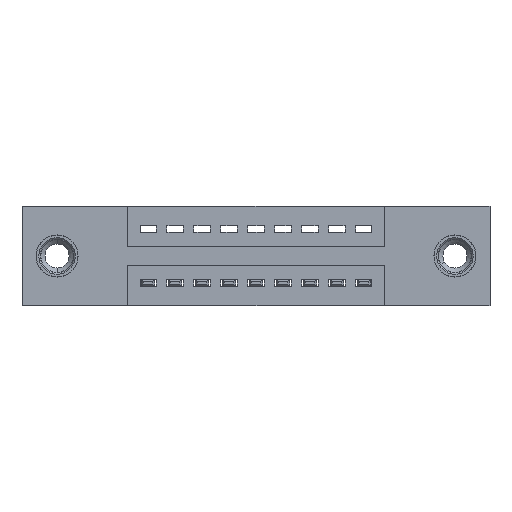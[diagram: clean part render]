
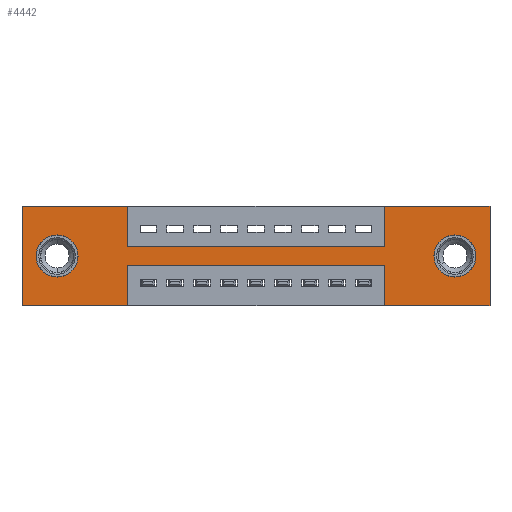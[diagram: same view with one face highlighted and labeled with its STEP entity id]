
A CAD part, front view. The second image highlights one B-rep face of the part: STEP entity #4442.
In plain terms, the highlighted planar face has unit normal (0, -1, 0).
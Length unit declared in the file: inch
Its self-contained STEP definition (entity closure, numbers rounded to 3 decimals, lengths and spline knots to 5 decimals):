
#3 = DIRECTION ( 'NONE',  ( 0., 1., 0. ) ) ;
#271 = ORIENTED_EDGE ( 'NONE', *, *, #3177, .T. ) ;
#413 = VERTEX_POINT ( 'NONE', #10230 ) ;
#442 = ORIENTED_EDGE ( 'NONE', *, *, #7183, .F. ) ;
#518 = CARTESIAN_POINT ( 'NONE',  ( 0.3925, 0., -0.37 ) ) ;
#746 = EDGE_CURVE ( 'NONE', #2080, #7335, #2838, .T. ) ;
#867 = DIRECTION ( 'NONE',  ( 1., 0., 0. ) ) ;
#895 = DIRECTION ( 'NONE',  ( 0., 0., -1. ) ) ;
#913 = ORIENTED_EDGE ( 'NONE', *, *, #9199, .F. ) ;
#1053 = CARTESIAN_POINT ( 'NONE',  ( 0., 0., 0. ) ) ;
#1136 = LINE ( 'NONE', #2850, #7727 ) ;
#1156 = CARTESIAN_POINT ( 'NONE',  ( 1.3425, 0., -0.15 ) ) ;
#1185 = ORIENTED_EDGE ( 'NONE', *, *, #5416, .F. ) ;
#1276 = CARTESIAN_POINT ( 'NONE',  ( 0.13, 0., -0.107 ) ) ;
#1354 = ORIENTED_EDGE ( 'NONE', *, *, #1799, .T. ) ;
#1493 = VECTOR ( 'NONE', #5650, 39.37008 ) ;
#1651 = DIRECTION ( 'NONE',  ( -1., 0., 0. ) ) ;
#1770 = CARTESIAN_POINT ( 'NONE',  ( 0.3925, 0., -0.22 ) ) ;
#1799 = EDGE_CURVE ( 'NONE', #8598, #413, #11335, .T. ) ;
#1884 = PLANE ( 'NONE',  #5999 ) ;
#1992 = DIRECTION ( 'NONE',  ( 1., 0., 0. ) ) ;
#2080 = VERTEX_POINT ( 'NONE', #1156 ) ;
#2261 = VERTEX_POINT ( 'NONE', #11005 ) ;
#2326 = CARTESIAN_POINT ( 'NONE',  ( 1.3425, 0., 0. ) ) ;
#2395 = EDGE_CURVE ( 'NONE', #7335, #11135, #8940, .T. ) ;
#2505 = ORIENTED_EDGE ( 'NONE', *, *, #2395, .F. ) ;
#2549 = DIRECTION ( 'NONE',  ( 0., 1., 0. ) ) ;
#2581 = AXIS2_PLACEMENT_3D ( 'NONE', #9398, #3808, #8330 ) ;
#2606 = VERTEX_POINT ( 'NONE', #7716 ) ;
#2838 = LINE ( 'NONE', #9803, #11215 ) ;
#2850 = CARTESIAN_POINT ( 'NONE',  ( 0.3925, 0., -0.37 ) ) ;
#2995 = CARTESIAN_POINT ( 'NONE',  ( 0.3925, 0., -0.15 ) ) ;
#3018 = CARTESIAN_POINT ( 'NONE',  ( 0.3925, 0., -0.22 ) ) ;
#3069 = VERTEX_POINT ( 'NONE', #1276 ) ;
#3105 = EDGE_CURVE ( 'NONE', #11135, #5520, #8944, .T. ) ;
#3177 = EDGE_CURVE ( 'NONE', #413, #8598, #6465, .T. ) ;
#3185 = ORIENTED_EDGE ( 'NONE', *, *, #3105, .F. ) ;
#3366 = CARTESIAN_POINT ( 'NONE',  ( 1.735, 0., -0.37 ) ) ;
#3478 = CARTESIAN_POINT ( 'NONE',  ( 1.3425, 0., -0.37 ) ) ;
#3547 = LINE ( 'NONE', #10758, #9218 ) ;
#3614 = ORIENTED_EDGE ( 'NONE', *, *, #11353, .F. ) ;
#3808 = DIRECTION ( 'NONE',  ( 0., 1., 0. ) ) ;
#3964 = DIRECTION ( 'NONE',  ( 0., 0., -1. ) ) ;
#3978 = EDGE_CURVE ( 'NONE', #4640, #4697, #9960, .T. ) ;
#4180 = AXIS2_PLACEMENT_3D ( 'NONE', #11761, #2549, #10909 ) ;
#4350 = VECTOR ( 'NONE', #1992, 39.37008 ) ;
#4442 = ADVANCED_FACE ( 'NONE', ( #7151, #11274, #8022 ), #1884, .T. ) ;
#4510 = ORIENTED_EDGE ( 'NONE', *, *, #11435, .F. ) ;
#4640 = VERTEX_POINT ( 'NONE', #8678 ) ;
#4697 = VERTEX_POINT ( 'NONE', #8754 ) ;
#4755 = CIRCLE ( 'NONE', #6246, 0.078 ) ;
#4995 = DIRECTION ( 'NONE',  ( 0., 1., 0. ) ) ;
#5001 = CARTESIAN_POINT ( 'NONE',  ( 0.3925, 0., 0. ) ) ;
#5041 = LINE ( 'NONE', #3478, #9084 ) ;
#5226 = CIRCLE ( 'NONE', #4180, 0.078 ) ;
#5318 = VECTOR ( 'NONE', #867, 39.37008 ) ;
#5327 = LINE ( 'NONE', #10306, #1493 ) ;
#5374 = DIRECTION ( 'NONE',  ( 0., 0., 1. ) ) ;
#5416 = EDGE_CURVE ( 'NONE', #8078, #8844, #10836, .T. ) ;
#5470 = VECTOR ( 'NONE', #11986, 39.37008 ) ;
#5520 = VERTEX_POINT ( 'NONE', #3366 ) ;
#5650 = DIRECTION ( 'NONE',  ( -1., 0., 0. ) ) ;
#5776 = CARTESIAN_POINT ( 'NONE',  ( 0.13, 0., -0.185 ) ) ;
#5940 = CARTESIAN_POINT ( 'NONE',  ( 0.13, 0., -0.263 ) ) ;
#5999 = AXIS2_PLACEMENT_3D ( 'NONE', #12231, #11164, #895 ) ;
#6017 = ORIENTED_EDGE ( 'NONE', *, *, #3978, .F. ) ;
#6239 = DIRECTION ( 'NONE',  ( 0., 0., -1. ) ) ;
#6246 = AXIS2_PLACEMENT_3D ( 'NONE', #5776, #3, #7465 ) ;
#6303 = VECTOR ( 'NONE', #3964, 39.37008 ) ;
#6465 = CIRCLE ( 'NONE', #6916, 0.078 ) ;
#6471 = ORIENTED_EDGE ( 'NONE', *, *, #7476, .T. ) ;
#6772 = VERTEX_POINT ( 'NONE', #7768 ) ;
#6908 = LINE ( 'NONE', #1770, #5470 ) ;
#6916 = AXIS2_PLACEMENT_3D ( 'NONE', #10548, #4995, #6239 ) ;
#7151 = FACE_BOUND ( 'NONE', #9599, .T. ) ;
#7183 = EDGE_CURVE ( 'NONE', #2261, #4640, #9575, .T. ) ;
#7335 = VERTEX_POINT ( 'NONE', #2326 ) ;
#7396 = EDGE_LOOP ( 'NONE', ( #8353, #4510, #3614, #8971, #3185, #2505, #11748, #9164, #6017, #442, #913, #1185 ) ) ;
#7465 = DIRECTION ( 'NONE',  ( 0., 0., 1. ) ) ;
#7476 = EDGE_CURVE ( 'NONE', #10048, #3069, #5226, .T. ) ;
#7692 = CARTESIAN_POINT ( 'NONE',  ( 1.735, 0., 0. ) ) ;
#7716 = CARTESIAN_POINT ( 'NONE',  ( 1.3425, 0., -0.22 ) ) ;
#7727 = VECTOR ( 'NONE', #11229, 39.37008 ) ;
#7768 = CARTESIAN_POINT ( 'NONE',  ( 1.3425, 0., -0.37 ) ) ;
#8022 = FACE_OUTER_BOUND ( 'NONE', #7396, .T. ) ;
#8078 = VERTEX_POINT ( 'NONE', #518 ) ;
#8310 = VECTOR ( 'NONE', #1651, 39.37008 ) ;
#8330 = DIRECTION ( 'NONE',  ( 0., 0., -1. ) ) ;
#8353 = ORIENTED_EDGE ( 'NONE', *, *, #10858, .F. ) ;
#8598 = VERTEX_POINT ( 'NONE', #12132 ) ;
#8678 = CARTESIAN_POINT ( 'NONE',  ( 0.3925, 0., 0. ) ) ;
#8725 = DIRECTION ( 'NONE',  ( 0., 0., 1. ) ) ;
#8744 = ORIENTED_EDGE ( 'NONE', *, *, #11204, .T. ) ;
#8754 = CARTESIAN_POINT ( 'NONE',  ( 0.3925, 0., -0.15 ) ) ;
#8844 = VERTEX_POINT ( 'NONE', #10524 ) ;
#8940 = LINE ( 'NONE', #12092, #5318 ) ;
#8944 = LINE ( 'NONE', #7692, #9237 ) ;
#8971 = ORIENTED_EDGE ( 'NONE', *, *, #11216, .F. ) ;
#9084 = VECTOR ( 'NONE', #5374, 39.37008 ) ;
#9164 = ORIENTED_EDGE ( 'NONE', *, *, #10276, .F. ) ;
#9199 = EDGE_CURVE ( 'NONE', #8844, #2261, #3547, .T. ) ;
#9218 = VECTOR ( 'NONE', #11686, 39.37008 ) ;
#9237 = VECTOR ( 'NONE', #11575, 39.37008 ) ;
#9398 = CARTESIAN_POINT ( 'NONE',  ( 1.605, 0., -0.185 ) ) ;
#9504 = VECTOR ( 'NONE', #10378, 39.37008 ) ;
#9575 = LINE ( 'NONE', #1053, #4350 ) ;
#9599 = EDGE_LOOP ( 'NONE', ( #271, #1354 ) ) ;
#9803 = CARTESIAN_POINT ( 'NONE',  ( 1.3425, 0., 0. ) ) ;
#9960 = LINE ( 'NONE', #5001, #6303 ) ;
#10048 = VERTEX_POINT ( 'NONE', #5940 ) ;
#10230 = CARTESIAN_POINT ( 'NONE',  ( 1.605, 0., -0.107 ) ) ;
#10276 = EDGE_CURVE ( 'NONE', #4697, #2080, #10725, .T. ) ;
#10306 = CARTESIAN_POINT ( 'NONE',  ( 0., 0., -0.37 ) ) ;
#10378 = DIRECTION ( 'NONE',  ( 1., 0., 0. ) ) ;
#10524 = CARTESIAN_POINT ( 'NONE',  ( 0., 0., -0.37 ) ) ;
#10548 = CARTESIAN_POINT ( 'NONE',  ( 1.605, 0., -0.185 ) ) ;
#10725 = LINE ( 'NONE', #2995, #9504 ) ;
#10758 = CARTESIAN_POINT ( 'NONE',  ( 0., 0., 0. ) ) ;
#10836 = LINE ( 'NONE', #10845, #8310 ) ;
#10845 = CARTESIAN_POINT ( 'NONE',  ( 0., 0., -0.37 ) ) ;
#10858 = EDGE_CURVE ( 'NONE', #11000, #8078, #1136, .T. ) ;
#10891 = EDGE_LOOP ( 'NONE', ( #8744, #6471 ) ) ;
#10909 = DIRECTION ( 'NONE',  ( 0., 0., 1. ) ) ;
#10977 = CARTESIAN_POINT ( 'NONE',  ( 1.735, 0., 0. ) ) ;
#11000 = VERTEX_POINT ( 'NONE', #3018 ) ;
#11005 = CARTESIAN_POINT ( 'NONE',  ( 0., 0., 0. ) ) ;
#11135 = VERTEX_POINT ( 'NONE', #10977 ) ;
#11164 = DIRECTION ( 'NONE',  ( 0., -1., 0. ) ) ;
#11204 = EDGE_CURVE ( 'NONE', #3069, #10048, #4755, .T. ) ;
#11215 = VECTOR ( 'NONE', #8725, 39.37008 ) ;
#11216 = EDGE_CURVE ( 'NONE', #5520, #6772, #5327, .T. ) ;
#11229 = DIRECTION ( 'NONE',  ( 0., 0., -1. ) ) ;
#11274 = FACE_BOUND ( 'NONE', #10891, .T. ) ;
#11335 = CIRCLE ( 'NONE', #2581, 0.078 ) ;
#11353 = EDGE_CURVE ( 'NONE', #6772, #2606, #5041, .T. ) ;
#11435 = EDGE_CURVE ( 'NONE', #2606, #11000, #6908, .T. ) ;
#11575 = DIRECTION ( 'NONE',  ( 0., 0., -1. ) ) ;
#11686 = DIRECTION ( 'NONE',  ( 0., 0., 1. ) ) ;
#11748 = ORIENTED_EDGE ( 'NONE', *, *, #746, .F. ) ;
#11761 = CARTESIAN_POINT ( 'NONE',  ( 0.13, 0., -0.185 ) ) ;
#11986 = DIRECTION ( 'NONE',  ( -1., 0., 0. ) ) ;
#12092 = CARTESIAN_POINT ( 'NONE',  ( 0., 0., 0. ) ) ;
#12132 = CARTESIAN_POINT ( 'NONE',  ( 1.605, 0., -0.263 ) ) ;
#12231 = CARTESIAN_POINT ( 'NONE',  ( 0., 0., -0.37 ) ) ;
